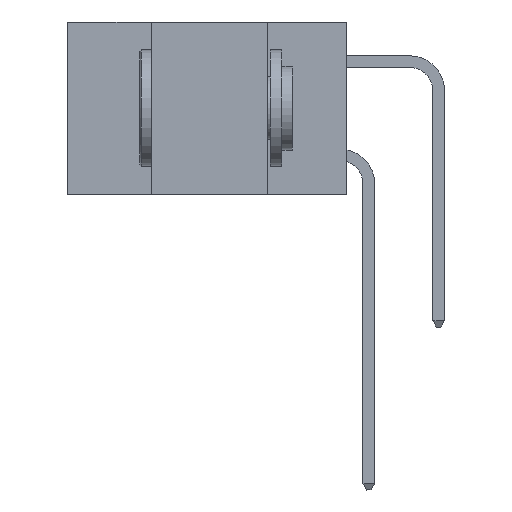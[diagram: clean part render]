
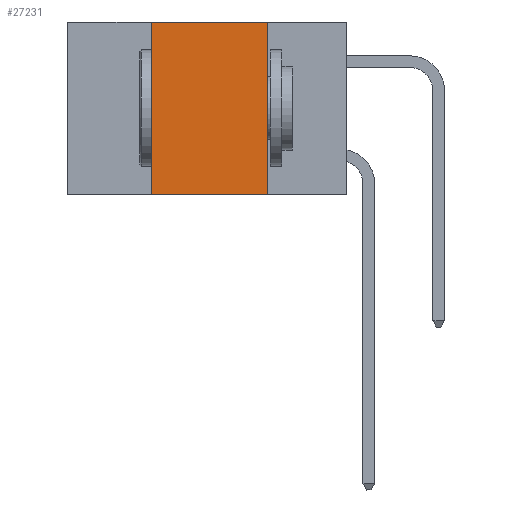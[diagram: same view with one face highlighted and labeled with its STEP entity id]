
A CAD part, left-side view. The second image highlights one B-rep face of the part: STEP entity #27231.
In plain terms, the highlighted planar face has unit normal (-1, 0, 0).
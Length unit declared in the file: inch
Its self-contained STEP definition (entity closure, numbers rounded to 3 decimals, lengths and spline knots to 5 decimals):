
#162 = CARTESIAN_POINT ( 'NONE',  ( 0., 0.6, 0. ) ) ;
#828 = LINE ( 'NONE', #21631, #28530 ) ;
#1272 = EDGE_CURVE ( 'NONE', #11237, #21893, #828, .T. ) ;
#1602 = DIRECTION ( 'NONE',  ( 0., -1., 0. ) ) ;
#3619 = ORIENTED_EDGE ( 'NONE', *, *, #23745, .F. ) ;
#4435 = LINE ( 'NONE', #15088, #19538 ) ;
#5130 = VERTEX_POINT ( 'NONE', #29157 ) ;
#6823 = VECTOR ( 'NONE', #14236, 39.37008 ) ;
#7004 = VECTOR ( 'NONE', #1602, 39.37008 ) ;
#7172 = DIRECTION ( 'NONE',  ( 0., 0., 1. ) ) ;
#10966 = AXIS2_PLACEMENT_3D ( 'NONE', #162, #18950, #21630 ) ;
#11237 = VERTEX_POINT ( 'NONE', #22122 ) ;
#13155 = PLANE ( 'NONE',  #10966 ) ;
#14236 = DIRECTION ( 'NONE',  ( 0., -1., 0. ) ) ;
#14352 = CARTESIAN_POINT ( 'NONE',  ( 0., 0.6, 0. ) ) ;
#15088 = CARTESIAN_POINT ( 'NONE',  ( 0., 0.42, 0. ) ) ;
#15951 = LINE ( 'NONE', #14352, #6823 ) ;
#16484 = EDGE_CURVE ( 'NONE', #5130, #11237, #15951, .T. ) ;
#17400 = VERTEX_POINT ( 'NONE', #26384 ) ;
#18726 = ORIENTED_EDGE ( 'NONE', *, *, #16484, .F. ) ;
#18950 = DIRECTION ( 'NONE',  ( 1., 0., 0. ) ) ;
#19364 = CARTESIAN_POINT ( 'NONE',  ( 0., 0.17, -0.37 ) ) ;
#19538 = VECTOR ( 'NONE', #7172, 39.37008 ) ;
#19579 = LINE ( 'NONE', #20454, #7004 ) ;
#19757 = EDGE_CURVE ( 'NONE', #17400, #21893, #19579, .T. ) ;
#20454 = CARTESIAN_POINT ( 'NONE',  ( 0., 0.6, -0.37 ) ) ;
#21569 = EDGE_LOOP ( 'NONE', ( #29967, #18726, #3619, #27017 ) ) ;
#21630 = DIRECTION ( 'NONE',  ( 0., 0., -1. ) ) ;
#21631 = CARTESIAN_POINT ( 'NONE',  ( 0., 0.17, 0. ) ) ;
#21893 = VERTEX_POINT ( 'NONE', #19364 ) ;
#22122 = CARTESIAN_POINT ( 'NONE',  ( 0., 0.17, 0. ) ) ;
#23745 = EDGE_CURVE ( 'NONE', #17400, #5130, #4435, .T. ) ;
#24437 = DIRECTION ( 'NONE',  ( 0., 0., -1. ) ) ;
#26384 = CARTESIAN_POINT ( 'NONE',  ( 0., 0.42, -0.37 ) ) ;
#27017 = ORIENTED_EDGE ( 'NONE', *, *, #19757, .T. ) ;
#27231 = ADVANCED_FACE ( 'NONE', ( #28070 ), #13155, .F. ) ;
#28070 = FACE_OUTER_BOUND ( 'NONE', #21569, .T. ) ;
#28530 = VECTOR ( 'NONE', #24437, 39.37008 ) ;
#29157 = CARTESIAN_POINT ( 'NONE',  ( 0., 0.42, 0. ) ) ;
#29967 = ORIENTED_EDGE ( 'NONE', *, *, #1272, .F. ) ;
